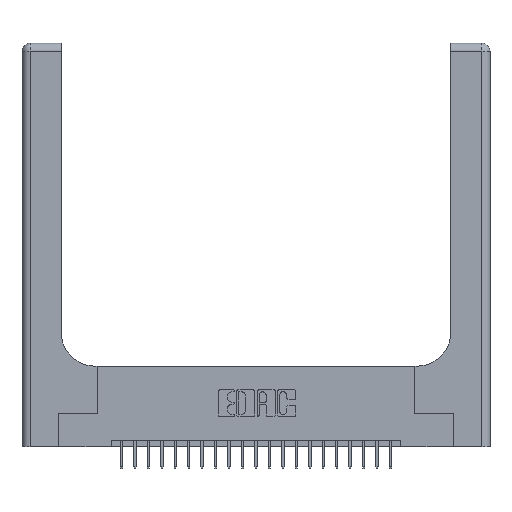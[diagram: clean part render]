
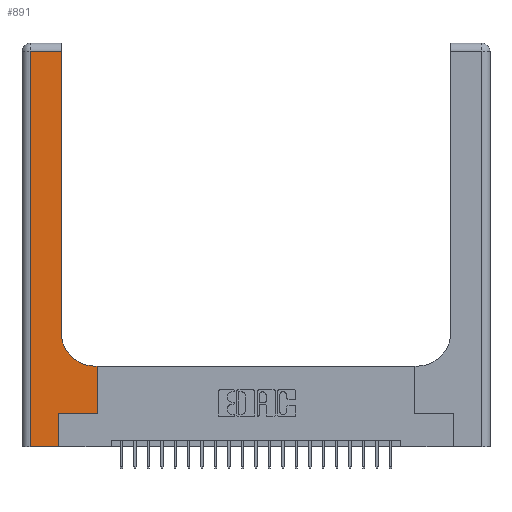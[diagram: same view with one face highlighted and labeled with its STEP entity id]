
A CAD part, top view. The second image highlights one B-rep face of the part: STEP entity #891.
In plain terms, the highlighted planar face has unit normal (0, 0, 1).
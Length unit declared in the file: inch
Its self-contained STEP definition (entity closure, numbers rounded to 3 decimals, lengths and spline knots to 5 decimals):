
#311 = VERTEX_POINT ( 'NONE', #6301 ) ;
#467 = DIRECTION ( 'NONE',  ( 0., 1., 0. ) ) ;
#752 = CARTESIAN_POINT ( 'NONE',  ( 0., 2.94, 0.37 ) ) ;
#891 = ADVANCED_FACE ( 'NONE', ( #7347 ), #22687, .F. ) ;
#1921 = CARTESIAN_POINT ( 'NONE',  ( 0.06, 2.94, 0.37 ) ) ;
#2416 = EDGE_CURVE ( 'NONE', #5847, #12327, #3586, .T. ) ;
#2923 = DIRECTION ( 'NONE',  ( 0., 0., -1. ) ) ;
#3475 = ORIENTED_EDGE ( 'NONE', *, *, #8901, .T. ) ;
#3524 = LINE ( 'NONE', #7642, #22414 ) ;
#3542 = DIRECTION ( 'NONE',  ( 1., 0., 0. ) ) ;
#3586 = LINE ( 'NONE', #7216, #23079 ) ;
#3790 = EDGE_CURVE ( 'NONE', #22897, #18836, #20335, .T. ) ;
#3939 = CARTESIAN_POINT ( 'NONE',  ( 0.06, 0., 0.37 ) ) ;
#4461 = LINE ( 'NONE', #16421, #14604 ) ;
#4723 = ORIENTED_EDGE ( 'NONE', *, *, #13531, .T. ) ;
#4789 = VECTOR ( 'NONE', #3542, 39.37008 ) ;
#5272 = CARTESIAN_POINT ( 'NONE',  ( 0.269, 0.25, 0.37 ) ) ;
#5518 = CARTESIAN_POINT ( 'NONE',  ( 0.2915, 2.94, 0.37 ) ) ;
#5539 = LINE ( 'NONE', #23201, #15059 ) ;
#5847 = VERTEX_POINT ( 'NONE', #8035 ) ;
#5904 = VECTOR ( 'NONE', #19176, 39.37008 ) ;
#5986 = CARTESIAN_POINT ( 'NONE',  ( 0.2915, 3., 0.37 ) ) ;
#6301 = CARTESIAN_POINT ( 'NONE',  ( 0.5415, 0.6, 0.37 ) ) ;
#6457 = VERTEX_POINT ( 'NONE', #1921 ) ;
#7091 = DIRECTION ( 'NONE',  ( 0., 1., 0. ) ) ;
#7216 = CARTESIAN_POINT ( 'NONE',  ( 0.269, 0., 0.37 ) ) ;
#7347 = FACE_OUTER_BOUND ( 'NONE', #22547, .T. ) ;
#7442 = ORIENTED_EDGE ( 'NONE', *, *, #17264, .T. ) ;
#7469 = ORIENTED_EDGE ( 'NONE', *, *, #3790, .T. ) ;
#7472 = CARTESIAN_POINT ( 'NONE',  ( 0.269, 0.25, 0.37 ) ) ;
#7642 = CARTESIAN_POINT ( 'NONE',  ( 0.2915, 0.6, 0.37 ) ) ;
#8035 = CARTESIAN_POINT ( 'NONE',  ( 0.269, 0., 0.37 ) ) ;
#8650 = ORIENTED_EDGE ( 'NONE', *, *, #13450, .T. ) ;
#8730 = VECTOR ( 'NONE', #16818, 39.37008 ) ;
#8901 = EDGE_CURVE ( 'NONE', #22925, #311, #3524, .T. ) ;
#9309 = EDGE_CURVE ( 'NONE', #6457, #15280, #4461, .T. ) ;
#9575 = DIRECTION ( 'NONE',  ( -1., 0., 0. ) ) ;
#10525 = CIRCLE ( 'NONE', #13529, 0.25 ) ;
#10803 = DIRECTION ( 'NONE',  ( 0., -1., 0. ) ) ;
#12327 = VERTEX_POINT ( 'NONE', #5272 ) ;
#13025 = EDGE_CURVE ( 'NONE', #12327, #20418, #13778, .T. ) ;
#13450 = EDGE_CURVE ( 'NONE', #311, #22897, #10525, .T. ) ;
#13529 = AXIS2_PLACEMENT_3D ( 'NONE', #14398, #2923, #16256 ) ;
#13531 = EDGE_CURVE ( 'NONE', #15280, #5847, #14333, .T. ) ;
#13778 = LINE ( 'NONE', #7472, #4789 ) ;
#13920 = EDGE_CURVE ( 'NONE', #18836, #6457, #21535, .T. ) ;
#14333 = LINE ( 'NONE', #14950, #8730 ) ;
#14398 = CARTESIAN_POINT ( 'NONE',  ( 0.5415, 0.85, 0.37 ) ) ;
#14604 = VECTOR ( 'NONE', #10803, 39.37008 ) ;
#14854 = ORIENTED_EDGE ( 'NONE', *, *, #2416, .T. ) ;
#14950 = CARTESIAN_POINT ( 'NONE',  ( 0., 0., 0.37 ) ) ;
#15059 = VECTOR ( 'NONE', #467, 39.37008 ) ;
#15280 = VERTEX_POINT ( 'NONE', #3939 ) ;
#16256 = DIRECTION ( 'NONE',  ( 1., 0., 0. ) ) ;
#16421 = CARTESIAN_POINT ( 'NONE',  ( 0.06, 3., 0.37 ) ) ;
#16818 = DIRECTION ( 'NONE',  ( 1., 0., 0. ) ) ;
#17264 = EDGE_CURVE ( 'NONE', #20418, #22925, #5539, .T. ) ;
#18036 = ORIENTED_EDGE ( 'NONE', *, *, #13920, .T. ) ;
#18836 = VERTEX_POINT ( 'NONE', #5518 ) ;
#19176 = DIRECTION ( 'NONE',  ( 0., 1., 0. ) ) ;
#20167 = CARTESIAN_POINT ( 'NONE',  ( 0.5585, 0.25, 0.37 ) ) ;
#20335 = LINE ( 'NONE', #5986, #5904 ) ;
#20383 = VECTOR ( 'NONE', #23624, 39.37008 ) ;
#20418 = VERTEX_POINT ( 'NONE', #20167 ) ;
#21535 = LINE ( 'NONE', #752, #20383 ) ;
#21766 = ORIENTED_EDGE ( 'NONE', *, *, #13025, .T. ) ;
#22137 = CARTESIAN_POINT ( 'NONE',  ( 0.5585, 0.6, 0.37 ) ) ;
#22414 = VECTOR ( 'NONE', #9575, 39.37008 ) ;
#22547 = EDGE_LOOP ( 'NONE', ( #7469, #18036, #22984, #4723, #14854, #21766, #7442, #3475, #8650 ) ) ;
#22687 = PLANE ( 'NONE',  #24407 ) ;
#22883 = DIRECTION ( 'NONE',  ( -1., 0., 0. ) ) ;
#22896 = DIRECTION ( 'NONE',  ( 0., 0., -1. ) ) ;
#22897 = VERTEX_POINT ( 'NONE', #23948 ) ;
#22925 = VERTEX_POINT ( 'NONE', #22137 ) ;
#22965 = CARTESIAN_POINT ( 'NONE',  ( 0., 3., 0.37 ) ) ;
#22984 = ORIENTED_EDGE ( 'NONE', *, *, #9309, .T. ) ;
#23079 = VECTOR ( 'NONE', #7091, 39.37008 ) ;
#23201 = CARTESIAN_POINT ( 'NONE',  ( 0.5585, 0.25, 0.37 ) ) ;
#23624 = DIRECTION ( 'NONE',  ( -1., 0., 0. ) ) ;
#23948 = CARTESIAN_POINT ( 'NONE',  ( 0.2915, 0.85, 0.37 ) ) ;
#24407 = AXIS2_PLACEMENT_3D ( 'NONE', #22965, #22896, #22883 ) ;
